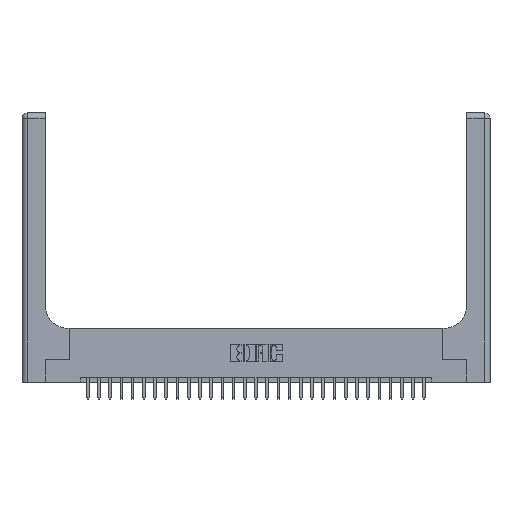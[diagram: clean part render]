
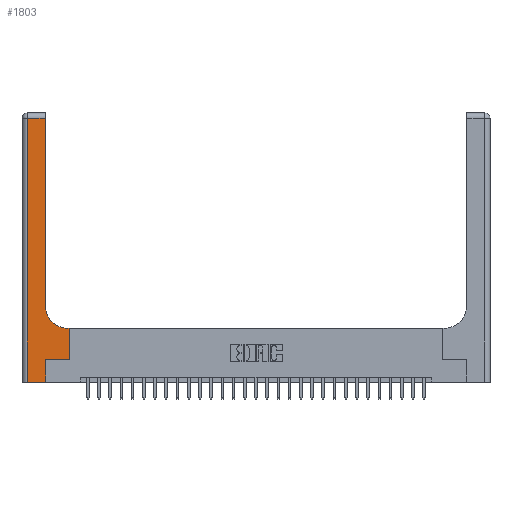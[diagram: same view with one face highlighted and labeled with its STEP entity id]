
A CAD part, top view. The second image highlights one B-rep face of the part: STEP entity #1803.
In plain terms, the highlighted planar face has unit normal (0, 0, 1).
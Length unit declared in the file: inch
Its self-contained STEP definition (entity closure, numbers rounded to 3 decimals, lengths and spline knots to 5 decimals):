
#8 = DIRECTION ( 'NONE',  ( 1., 0., 0. ) ) ;
#1755 = ORIENTED_EDGE ( 'NONE', *, *, #17738, .T. ) ;
#1803 = ADVANCED_FACE ( 'NONE', ( #12190 ), #26552, .F. ) ;
#2050 = CARTESIAN_POINT ( 'NONE',  ( 0.528, 0.6, 0.37 ) ) ;
#3438 = VECTOR ( 'NONE', #12100, 39.37008 ) ;
#3526 = ORIENTED_EDGE ( 'NONE', *, *, #10008, .T. ) ;
#3771 = VECTOR ( 'NONE', #10077, 39.37008 ) ;
#4261 = LINE ( 'NONE', #11430, #4922 ) ;
#4800 = ORIENTED_EDGE ( 'NONE', *, *, #10634, .T. ) ;
#4837 = LINE ( 'NONE', #14684, #15945 ) ;
#4922 = VECTOR ( 'NONE', #17640, 39.37008 ) ;
#5031 = CARTESIAN_POINT ( 'NONE',  ( 0.26, 2.94, 0.37 ) ) ;
#6252 = VERTEX_POINT ( 'NONE', #12609 ) ;
#6271 = CARTESIAN_POINT ( 'NONE',  ( 0.51, 0.85, 0.37 ) ) ;
#7057 = DIRECTION ( 'NONE',  ( 0., 1., 0. ) ) ;
#7070 = ORIENTED_EDGE ( 'NONE', *, *, #24236, .T. ) ;
#7706 = VECTOR ( 'NONE', #7057, 39.37008 ) ;
#7912 = CARTESIAN_POINT ( 'NONE',  ( 0.26, 0.6, 0.37 ) ) ;
#7982 = CARTESIAN_POINT ( 'NONE',  ( 0., 2.94, 0.37 ) ) ;
#8004 = AXIS2_PLACEMENT_3D ( 'NONE', #14284, #26828, #20433 ) ;
#8036 = CIRCLE ( 'NONE', #11915, 0.25 ) ;
#8076 = CARTESIAN_POINT ( 'NONE',  ( 0.51, 0.6, 0.37 ) ) ;
#8205 = DIRECTION ( 'NONE',  ( 0., 0., -1. ) ) ;
#8444 = VERTEX_POINT ( 'NONE', #12036 ) ;
#9018 = ORIENTED_EDGE ( 'NONE', *, *, #24742, .T. ) ;
#9683 = LINE ( 'NONE', #7982, #3438 ) ;
#10008 = EDGE_CURVE ( 'NONE', #8444, #21942, #22171, .T. ) ;
#10037 = EDGE_CURVE ( 'NONE', #17948, #12845, #4837, .T. ) ;
#10077 = DIRECTION ( 'NONE',  ( 0., 1., 0. ) ) ;
#10104 = EDGE_LOOP ( 'NONE', ( #1755, #13192, #17472, #4800, #25026, #3526, #14152, #9018, #7070 ) ) ;
#10171 = CARTESIAN_POINT ( 'NONE',  ( 0.528, 0.25, 0.37 ) ) ;
#10634 = EDGE_CURVE ( 'NONE', #12845, #6252, #24422, .T. ) ;
#11430 = CARTESIAN_POINT ( 'NONE',  ( 0.26, 3., 0.37 ) ) ;
#11915 = AXIS2_PLACEMENT_3D ( 'NONE', #6271, #8205, #8 ) ;
#12036 = CARTESIAN_POINT ( 'NONE',  ( 0.265, 0.25, 0.37 ) ) ;
#12100 = DIRECTION ( 'NONE',  ( -1., 0., 0. ) ) ;
#12190 = FACE_OUTER_BOUND ( 'NONE', #10104, .T. ) ;
#12212 = DIRECTION ( 'NONE',  ( 1., 0., 0. ) ) ;
#12320 = EDGE_CURVE ( 'NONE', #6252, #8444, #22090, .T. ) ;
#12510 = CARTESIAN_POINT ( 'NONE',  ( 0.06, 2.94, 0.37 ) ) ;
#12609 = CARTESIAN_POINT ( 'NONE',  ( 0.265, 0., 0.37 ) ) ;
#12845 = VERTEX_POINT ( 'NONE', #25139 ) ;
#13192 = ORIENTED_EDGE ( 'NONE', *, *, #23954, .T. ) ;
#14152 = ORIENTED_EDGE ( 'NONE', *, *, #23908, .T. ) ;
#14188 = CARTESIAN_POINT ( 'NONE',  ( 0., 0., 0.37 ) ) ;
#14284 = CARTESIAN_POINT ( 'NONE',  ( 0., 3., 0.37 ) ) ;
#14542 = VERTEX_POINT ( 'NONE', #2050 ) ;
#14592 = CARTESIAN_POINT ( 'NONE',  ( 0.26, 0.85, 0.37 ) ) ;
#14684 = CARTESIAN_POINT ( 'NONE',  ( 0.06, 3., 0.37 ) ) ;
#14865 = LINE ( 'NONE', #10171, #3771 ) ;
#15360 = CARTESIAN_POINT ( 'NONE',  ( 0.265, 0., 0.37 ) ) ;
#15917 = VECTOR ( 'NONE', #12212, 39.37008 ) ;
#15945 = VECTOR ( 'NONE', #19160, 39.37008 ) ;
#16603 = VECTOR ( 'NONE', #25365, 39.37008 ) ;
#16798 = LINE ( 'NONE', #7912, #24660 ) ;
#17472 = ORIENTED_EDGE ( 'NONE', *, *, #10037, .T. ) ;
#17640 = DIRECTION ( 'NONE',  ( 0., 1., 0. ) ) ;
#17738 = EDGE_CURVE ( 'NONE', #17962, #20802, #4261, .T. ) ;
#17948 = VERTEX_POINT ( 'NONE', #12510 ) ;
#17962 = VERTEX_POINT ( 'NONE', #14592 ) ;
#18410 = DIRECTION ( 'NONE',  ( -1., 0., 0. ) ) ;
#19160 = DIRECTION ( 'NONE',  ( 0., -1., 0. ) ) ;
#20433 = DIRECTION ( 'NONE',  ( -1., 0., 0. ) ) ;
#20570 = VERTEX_POINT ( 'NONE', #8076 ) ;
#20802 = VERTEX_POINT ( 'NONE', #5031 ) ;
#21163 = CARTESIAN_POINT ( 'NONE',  ( 0.265, 0.25, 0.37 ) ) ;
#21942 = VERTEX_POINT ( 'NONE', #24968 ) ;
#22090 = LINE ( 'NONE', #15360, #7706 ) ;
#22171 = LINE ( 'NONE', #21163, #16603 ) ;
#23908 = EDGE_CURVE ( 'NONE', #21942, #14542, #14865, .T. ) ;
#23954 = EDGE_CURVE ( 'NONE', #20802, #17948, #9683, .T. ) ;
#24236 = EDGE_CURVE ( 'NONE', #20570, #17962, #8036, .T. ) ;
#24422 = LINE ( 'NONE', #14188, #15917 ) ;
#24660 = VECTOR ( 'NONE', #18410, 39.37008 ) ;
#24742 = EDGE_CURVE ( 'NONE', #14542, #20570, #16798, .T. ) ;
#24968 = CARTESIAN_POINT ( 'NONE',  ( 0.528, 0.25, 0.37 ) ) ;
#25026 = ORIENTED_EDGE ( 'NONE', *, *, #12320, .T. ) ;
#25139 = CARTESIAN_POINT ( 'NONE',  ( 0.06, 0., 0.37 ) ) ;
#25365 = DIRECTION ( 'NONE',  ( 1., 0., 0. ) ) ;
#26552 = PLANE ( 'NONE',  #8004 ) ;
#26828 = DIRECTION ( 'NONE',  ( 0., 0., -1. ) ) ;
